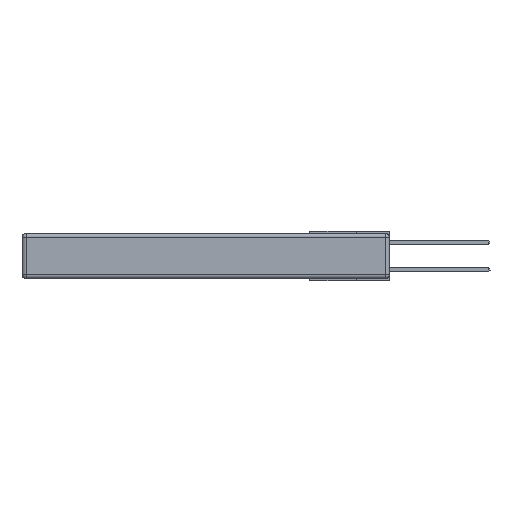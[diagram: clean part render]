
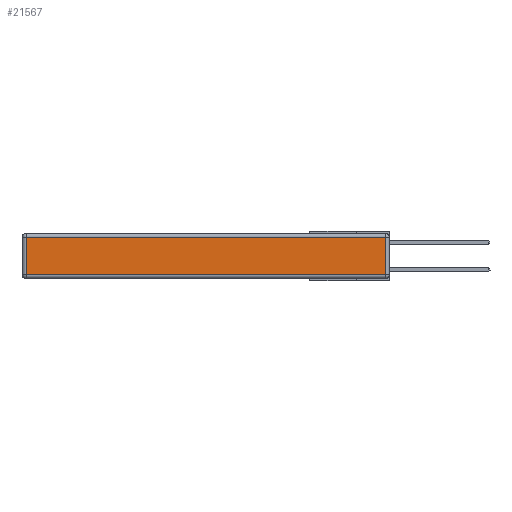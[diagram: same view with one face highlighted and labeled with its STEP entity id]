
A CAD part, left-side view. The second image highlights one B-rep face of the part: STEP entity #21567.
In plain terms, the highlighted planar face has unit normal (-1, 0, 0).
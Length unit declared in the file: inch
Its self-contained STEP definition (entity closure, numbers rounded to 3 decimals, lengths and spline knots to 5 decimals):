
#1269 = LINE ( 'NONE', #27541, #17942 ) ;
#1844 = VERTEX_POINT ( 'NONE', #27320 ) ;
#1880 = ORIENTED_EDGE ( 'NONE', *, *, #5557, .T. ) ;
#2210 = DIRECTION ( 'NONE',  ( 0., 1., 0. ) ) ;
#2374 = DIRECTION ( 'NONE',  ( -1., 0., 0. ) ) ;
#2476 = CARTESIAN_POINT ( 'NONE',  ( 0., 0., -0.343 ) ) ;
#3191 = VERTEX_POINT ( 'NONE', #8179 ) ;
#3384 = ORIENTED_EDGE ( 'NONE', *, *, #5689, .T. ) ;
#3631 = LINE ( 'NONE', #9140, #26361 ) ;
#4933 = VECTOR ( 'NONE', #24343, 39.37008 ) ;
#5557 = EDGE_CURVE ( 'NONE', #3191, #1844, #1269, .T. ) ;
#5689 = EDGE_CURVE ( 'NONE', #17503, #11350, #6287, .T. ) ;
#6287 = LINE ( 'NONE', #19992, #4933 ) ;
#7265 = ORIENTED_EDGE ( 'NONE', *, *, #16114, .T. ) ;
#8179 = CARTESIAN_POINT ( 'NONE',  ( 0., 2.72, -0.03 ) ) ;
#8877 = PLANE ( 'NONE',  #21888 ) ;
#9140 = CARTESIAN_POINT ( 'NONE',  ( 0., 0., -0.313 ) ) ;
#10094 = LINE ( 'NONE', #20993, #12463 ) ;
#11350 = VERTEX_POINT ( 'NONE', #23009 ) ;
#11820 = EDGE_CURVE ( 'NONE', #11350, #3191, #10094, .T. ) ;
#12463 = VECTOR ( 'NONE', #2210, 39.37008 ) ;
#15558 = DIRECTION ( 'NONE',  ( 0., 0., 1. ) ) ;
#16114 = EDGE_CURVE ( 'NONE', #1844, #17503, #3631, .T. ) ;
#17503 = VERTEX_POINT ( 'NONE', #20215 ) ;
#17942 = VECTOR ( 'NONE', #18978, 39.37008 ) ;
#18328 = DIRECTION ( 'NONE',  ( 0., -1., 0. ) ) ;
#18715 = FACE_OUTER_BOUND ( 'NONE', #23070, .T. ) ;
#18978 = DIRECTION ( 'NONE',  ( 0., 0., -1. ) ) ;
#19992 = CARTESIAN_POINT ( 'NONE',  ( 0., 0.03, -0.343 ) ) ;
#20215 = CARTESIAN_POINT ( 'NONE',  ( 0., 0.03, -0.313 ) ) ;
#20993 = CARTESIAN_POINT ( 'NONE',  ( 0., 2.75, -0.03 ) ) ;
#21555 = ORIENTED_EDGE ( 'NONE', *, *, #11820, .T. ) ;
#21567 = ADVANCED_FACE ( 'NONE', ( #18715 ), #8877, .T. ) ;
#21888 = AXIS2_PLACEMENT_3D ( 'NONE', #2476, #2374, #15558 ) ;
#23009 = CARTESIAN_POINT ( 'NONE',  ( 0., 0.03, -0.03 ) ) ;
#23070 = EDGE_LOOP ( 'NONE', ( #7265, #3384, #21555, #1880 ) ) ;
#24343 = DIRECTION ( 'NONE',  ( 0., 0., 1. ) ) ;
#26361 = VECTOR ( 'NONE', #18328, 39.37008 ) ;
#27320 = CARTESIAN_POINT ( 'NONE',  ( 0., 2.72, -0.313 ) ) ;
#27541 = CARTESIAN_POINT ( 'NONE',  ( 0., 2.72, -0.343 ) ) ;
